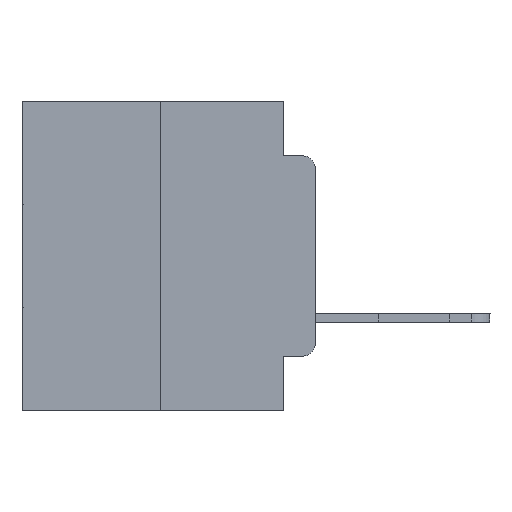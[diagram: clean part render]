
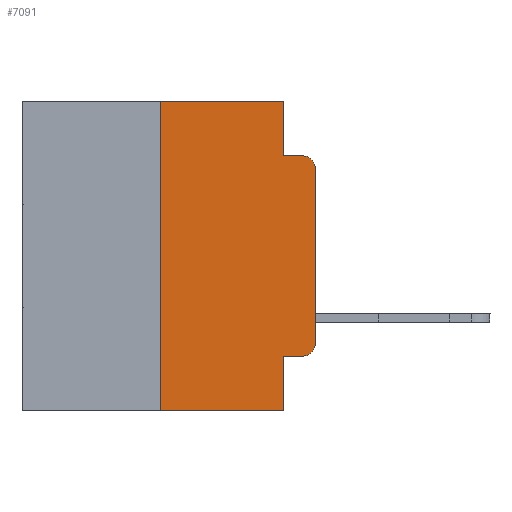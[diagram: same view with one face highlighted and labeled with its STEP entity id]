
A CAD part, left-side view. The second image highlights one B-rep face of the part: STEP entity #7091.
In plain terms, the highlighted planar face has unit normal (-1, 0, 0).
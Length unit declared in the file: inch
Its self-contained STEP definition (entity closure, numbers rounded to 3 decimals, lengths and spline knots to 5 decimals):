
#386 = VECTOR ( 'NONE', #7531, 39.37008 ) ;
#1099 = ORIENTED_EDGE ( 'NONE', *, *, #7407, .T. ) ;
#1124 = CARTESIAN_POINT ( 'NONE',  ( 0., 0.051, 0. ) ) ;
#1590 = VECTOR ( 'NONE', #15994, 39.37008 ) ;
#1760 = ORIENTED_EDGE ( 'NONE', *, *, #17610, .T. ) ;
#1801 = LINE ( 'NONE', #12227, #12867 ) ;
#2610 = DIRECTION ( 'NONE',  ( -1., 0., 0. ) ) ;
#2646 = ORIENTED_EDGE ( 'NONE', *, *, #9736, .F. ) ;
#3103 = ORIENTED_EDGE ( 'NONE', *, *, #14863, .T. ) ;
#4180 = DIRECTION ( 'NONE',  ( -1., 0., 0. ) ) ;
#4230 = CARTESIAN_POINT ( 'NONE',  ( 0., 0.25, 0. ) ) ;
#4288 = EDGE_CURVE ( 'NONE', #21127, #19082, #4784, .T. ) ;
#4351 = DIRECTION ( 'NONE',  ( 0., 0., -1. ) ) ;
#4469 = CARTESIAN_POINT ( 'NONE',  ( 0., 0.02, -0.3915 ) ) ;
#4607 = DIRECTION ( 'NONE',  ( 1., 0., 0. ) ) ;
#4784 = LINE ( 'NONE', #10520, #20322 ) ;
#5144 = VECTOR ( 'NONE', #5601, 39.37008 ) ;
#5601 = DIRECTION ( 'NONE',  ( 0., -1., 0. ) ) ;
#5641 = EDGE_CURVE ( 'NONE', #21127, #14446, #1801, .T. ) ;
#6165 = CARTESIAN_POINT ( 'NONE',  ( 0., 0.051, -0.5 ) ) ;
#6407 = CARTESIAN_POINT ( 'NONE',  ( 0., 0.473, -0.5 ) ) ;
#6773 = EDGE_CURVE ( 'NONE', #16368, #11245, #20000, .T. ) ;
#6816 = ORIENTED_EDGE ( 'NONE', *, *, #5641, .F. ) ;
#6902 = VECTOR ( 'NONE', #24311, 39.37008 ) ;
#7091 = ADVANCED_FACE ( 'NONE', ( #13031 ), #14780, .F. ) ;
#7407 = EDGE_CURVE ( 'NONE', #7935, #11245, #20853, .T. ) ;
#7531 = DIRECTION ( 'NONE',  ( 0., 0., 1. ) ) ;
#7599 = LINE ( 'NONE', #15784, #5144 ) ;
#7860 = LINE ( 'NONE', #6407, #22904 ) ;
#7935 = VERTEX_POINT ( 'NONE', #25113 ) ;
#8400 = EDGE_CURVE ( 'NONE', #19255, #7935, #13945, .T. ) ;
#8420 = CARTESIAN_POINT ( 'NONE',  ( 0., 0.051, -0.4115 ) ) ;
#8435 = VERTEX_POINT ( 'NONE', #1124 ) ;
#8672 = ORIENTED_EDGE ( 'NONE', *, *, #8400, .T. ) ;
#9736 = EDGE_CURVE ( 'NONE', #12835, #8435, #7599, .T. ) ;
#10199 = AXIS2_PLACEMENT_3D ( 'NONE', #4469, #2610, #4351 ) ;
#10520 = CARTESIAN_POINT ( 'NONE',  ( 0., 0.051, -0.4115 ) ) ;
#10862 = LINE ( 'NONE', #19030, #14190 ) ;
#11245 = VERTEX_POINT ( 'NONE', #20984 ) ;
#11583 = CARTESIAN_POINT ( 'NONE',  ( 0., 0.051, -0.0885 ) ) ;
#11692 = ORIENTED_EDGE ( 'NONE', *, *, #6773, .F. ) ;
#12227 = CARTESIAN_POINT ( 'NONE',  ( 0., 0.051, 0. ) ) ;
#12770 = DIRECTION ( 'NONE',  ( 0., 0., -1. ) ) ;
#12835 = VERTEX_POINT ( 'NONE', #4230 ) ;
#12867 = VECTOR ( 'NONE', #13972, 39.37008 ) ;
#13031 = FACE_OUTER_BOUND ( 'NONE', #19550, .T. ) ;
#13315 = CARTESIAN_POINT ( 'NONE',  ( 0., 0.02, -0.4115 ) ) ;
#13945 = LINE ( 'NONE', #23730, #386 ) ;
#13972 = DIRECTION ( 'NONE',  ( 0., 0., -1. ) ) ;
#14002 = ORIENTED_EDGE ( 'NONE', *, *, #22517, .F. ) ;
#14190 = VECTOR ( 'NONE', #14888, 39.37008 ) ;
#14435 = DIRECTION ( 'NONE',  ( 0., -1., 0. ) ) ;
#14446 = VERTEX_POINT ( 'NONE', #6165 ) ;
#14780 = PLANE ( 'NONE',  #22524 ) ;
#14863 = EDGE_CURVE ( 'NONE', #25437, #14446, #7860, .T. ) ;
#14888 = DIRECTION ( 'NONE',  ( 0., 0., -1. ) ) ;
#15363 = CIRCLE ( 'NONE', #10199, 0.02 ) ;
#15784 = CARTESIAN_POINT ( 'NONE',  ( 0., 0.473, 0. ) ) ;
#15994 = DIRECTION ( 'NONE',  ( 0., -1., 0. ) ) ;
#16173 = CARTESIAN_POINT ( 'NONE',  ( 0., 0.25, 0. ) ) ;
#16368 = VERTEX_POINT ( 'NONE', #17508 ) ;
#16971 = ORIENTED_EDGE ( 'NONE', *, *, #21509, .F. ) ;
#17508 = CARTESIAN_POINT ( 'NONE',  ( 0., 0.051, -0.0885 ) ) ;
#17610 = EDGE_CURVE ( 'NONE', #19082, #19255, #15363, .T. ) ;
#18908 = CARTESIAN_POINT ( 'NONE',  ( 0., 0., -0.3915 ) ) ;
#19030 = CARTESIAN_POINT ( 'NONE',  ( 0., 0.051, 0. ) ) ;
#19082 = VERTEX_POINT ( 'NONE', #13315 ) ;
#19255 = VERTEX_POINT ( 'NONE', #18908 ) ;
#19550 = EDGE_LOOP ( 'NONE', ( #8672, #1099, #11692, #14002, #2646, #16971, #3103, #6816, #25848, #1760 ) ) ;
#20000 = LINE ( 'NONE', #11583, #1590 ) ;
#20322 = VECTOR ( 'NONE', #22836, 39.37008 ) ;
#20437 = AXIS2_PLACEMENT_3D ( 'NONE', #26374, #4180, #24239 ) ;
#20853 = CIRCLE ( 'NONE', #20437, 0.02 ) ;
#20984 = CARTESIAN_POINT ( 'NONE',  ( 0., 0.02, -0.0885 ) ) ;
#21127 = VERTEX_POINT ( 'NONE', #8420 ) ;
#21509 = EDGE_CURVE ( 'NONE', #25437, #12835, #22578, .T. ) ;
#22517 = EDGE_CURVE ( 'NONE', #8435, #16368, #10862, .T. ) ;
#22524 = AXIS2_PLACEMENT_3D ( 'NONE', #22931, #4607, #12770 ) ;
#22578 = LINE ( 'NONE', #16173, #6902 ) ;
#22836 = DIRECTION ( 'NONE',  ( 0., -1., 0. ) ) ;
#22904 = VECTOR ( 'NONE', #14435, 39.37008 ) ;
#22931 = CARTESIAN_POINT ( 'NONE',  ( 0., 0.473, 0. ) ) ;
#23730 = CARTESIAN_POINT ( 'NONE',  ( 0., 0., 0. ) ) ;
#24239 = DIRECTION ( 'NONE',  ( 0., 0., -1. ) ) ;
#24311 = DIRECTION ( 'NONE',  ( 0., 0., 1. ) ) ;
#24620 = CARTESIAN_POINT ( 'NONE',  ( 0., 0.25, -0.5 ) ) ;
#25113 = CARTESIAN_POINT ( 'NONE',  ( 0., 0., -0.1085 ) ) ;
#25437 = VERTEX_POINT ( 'NONE', #24620 ) ;
#25848 = ORIENTED_EDGE ( 'NONE', *, *, #4288, .T. ) ;
#26374 = CARTESIAN_POINT ( 'NONE',  ( 0., 0.02, -0.1085 ) ) ;
